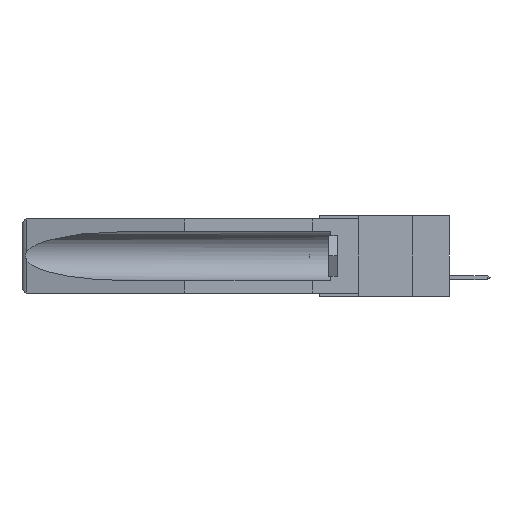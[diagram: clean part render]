
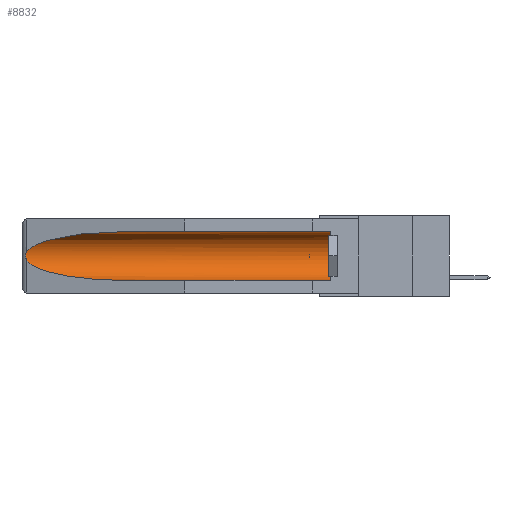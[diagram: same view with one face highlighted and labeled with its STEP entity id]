
A CAD part, left-side view. The second image highlights one B-rep face of the part: STEP entity #8832.
In plain terms, the highlighted cylindrical face has radius 2.857 mm (diameter 5.715 mm), a partial arc.
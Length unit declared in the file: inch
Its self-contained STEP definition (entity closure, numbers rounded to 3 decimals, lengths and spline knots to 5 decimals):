
#994 = ORIENTED_EDGE ( 'NONE', *, *, #16064, .T. ) ;
#1166 = CARTESIAN_POINT ( 'NONE',  ( 0.21114, 1.30732, -0.284 ) ) ;
#1522 = CARTESIAN_POINT ( 'NONE',  ( 0.2675, 1.53308, -0.17534 ) ) ;
#3514 = ORIENTED_EDGE ( 'NONE', *, *, #29029, .T. ) ;
#3515 = CARTESIAN_POINT ( 'NONE',  ( 0.25451, 1.48313, -0.24835 ) ) ;
#3572 = CARTESIAN_POINT ( 'NONE',  ( 0.26537, 1.52718, -0.14972 ) ) ;
#3663 = VERTEX_POINT ( 'NONE', #31776 ) ;
#4320 = CARTESIAN_POINT ( 'NONE',  ( 0.2675, 1.53308, -0.16763 ) ) ;
#4430 = CARTESIAN_POINT ( 'NONE',  ( 0.26597, 1.5296, -0.19026 ) ) ;
#5067 = CARTESIAN_POINT ( 'NONE',  ( 0.155, -0.30754, -0.1715 ) ) ;
#6015 = CARTESIAN_POINT ( 'NONE',  ( 0.155, 1.07973, -0.059 ) ) ;
#6191 = LINE ( 'NONE', #8923, #11631 ) ;
#6878 = CARTESIAN_POINT ( 'NONE',  ( 0.26537, 1.52718, -0.19328 ) ) ;
#7619 = CYLINDRICAL_SURFACE ( 'NONE', #25311, 0.1125 ) ;
#8011 = ORIENTED_EDGE ( 'NONE', *, *, #21563, .F. ) ;
#8250 = CARTESIAN_POINT ( 'NONE',  ( 0.155, 0.126, -0.284 ) ) ;
#8832 = ADVANCED_FACE ( 'NONE', ( #28910 ), #7619, .F. ) ;
#8923 = CARTESIAN_POINT ( 'NONE',  ( 0.155, -0.30754, -0.059 ) ) ;
#9689 = CARTESIAN_POINT ( 'NONE',  ( 0.2673, 1.5327, -0.16383 ) ) ;
#10034 = CARTESIAN_POINT ( 'NONE',  ( 0.26654, 1.53092, -0.15636 ) ) ;
#10948 = CARTESIAN_POINT ( 'NONE',  ( 0.155, -0.30754, -0.284 ) ) ;
#11548 = VERTEX_POINT ( 'NONE', #20221 ) ;
#11631 = VECTOR ( 'NONE', #27247, 39.37008 ) ;
#13234 = B_SPLINE_CURVE_WITH_KNOTS ( 'NONE', 3,
 ( #17983, #25590, #10034, #9689, #4320, #1522, #20552, #17507, #4430, #6878 ),
 .UNSPECIFIED., .F., .F.,
 ( 4, 2, 2, 2, 4 ),
 ( 0., 0.00029, 0.00058, 0.00087, 0.00117 ),
 .UNSPECIFIED. ) ;
#13338 = DIRECTION ( 'NONE',  ( 0., 1., 0. ) ) ;
#13407 = DIRECTION ( 'NONE',  ( 0., 1., 0. ) ) ;
#14192 = CARTESIAN_POINT ( 'NONE',  ( 0.21114, 1.30732, -0.059 ) ) ;
#14549 = VECTOR ( 'NONE', #13407, 39.37008 ) ;
#14840 = CARTESIAN_POINT ( 'NONE',  ( 0.155, 1.07973, -0.284 ) ) ;
#15568 = VERTEX_POINT ( 'NONE', #8250 ) ;
#15584 = DIRECTION ( 'NONE',  ( 0., -1., 0. ) ) ;
#16064 = EDGE_CURVE ( 'NONE', #15568, #30093, #21509, .T. ) ;
#16155 = ORIENTED_EDGE ( 'NONE', *, *, #25836, .T. ) ;
#16664 = LINE ( 'NONE', #10948, #14549 ) ;
#17188 = CARTESIAN_POINT ( 'NONE',  ( 0.26537, 1.52718, -0.19328 ) ) ;
#17507 = CARTESIAN_POINT ( 'NONE',  ( 0.26655, 1.53094, -0.18657 ) ) ;
#17831 = VERTEX_POINT ( 'NONE', #32476 ) ;
#17983 = CARTESIAN_POINT ( 'NONE',  ( 0.26537, 1.52718, -0.14972 ) ) ;
#19095 = EDGE_LOOP ( 'NONE', ( #16155, #22995, #3514, #8011, #994, #25543 ) ) ;
#20221 = CARTESIAN_POINT ( 'NONE',  ( 0.26537, 1.52718, -0.19328 ) ) ;
#20301 = CARTESIAN_POINT ( 'NONE',  ( 0.155, 1.07973, -0.059 ) ) ;
#20552 = CARTESIAN_POINT ( 'NONE',  ( 0.2673, 1.53269, -0.17917 ) ) ;
#21509 = CIRCLE ( 'NONE', #23183, 0.1125 ) ;
#21563 = EDGE_CURVE ( 'NONE', #15568, #17831, #16664, .T. ) ;
#22122 = CARTESIAN_POINT ( 'NONE',  ( 0.25451, 1.48313, -0.09465 ) ) ;
#22635 =( BOUNDED_CURVE ( )  B_SPLINE_CURVE ( 3, ( #17188, #3515, #1166, #14840 ),
 .UNSPECIFIED., .F., .F. ) 
 B_SPLINE_CURVE_WITH_KNOTS ( ( 4, 4 ),
 ( 0.1948, 1.5708 ),
 .UNSPECIFIED. ) 
 CURVE ( )  GEOMETRIC_REPRESENTATION_ITEM ( )  RATIONAL_B_SPLINE_CURVE ( ( 1., 0.848, 0.848, 1. ) ) 
 REPRESENTATION_ITEM ( '' )  );
#22995 = ORIENTED_EDGE ( 'NONE', *, *, #29917, .T. ) ;
#23183 = AXIS2_PLACEMENT_3D ( 'NONE', #31542, #15584, #34198 ) ;
#23717 = VERTEX_POINT ( 'NONE', #20301 ) ;
#23856 = DIRECTION ( 'NONE',  ( 0., 0., 1. ) ) ;
#25311 = AXIS2_PLACEMENT_3D ( 'NONE', #5067, #13338, #23856 ) ;
#25543 = ORIENTED_EDGE ( 'NONE', *, *, #28626, .T. ) ;
#25590 = CARTESIAN_POINT ( 'NONE',  ( 0.26597, 1.52961, -0.15275 ) ) ;
#25836 = EDGE_CURVE ( 'NONE', #23717, #3663, #32432, .T. ) ;
#27247 = DIRECTION ( 'NONE',  ( 0., 1., 0. ) ) ;
#28626 = EDGE_CURVE ( 'NONE', #30093, #23717, #6191, .T. ) ;
#28910 = FACE_OUTER_BOUND ( 'NONE', #19095, .T. ) ;
#28928 = CARTESIAN_POINT ( 'NONE',  ( 0.155, 0.126, -0.059 ) ) ;
#29029 = EDGE_CURVE ( 'NONE', #11548, #17831, #22635, .T. ) ;
#29917 = EDGE_CURVE ( 'NONE', #3663, #11548, #13234, .T. ) ;
#30093 = VERTEX_POINT ( 'NONE', #28928 ) ;
#31542 = CARTESIAN_POINT ( 'NONE',  ( 0.155, 0.126, -0.1715 ) ) ;
#31776 = CARTESIAN_POINT ( 'NONE',  ( 0.26537, 1.52718, -0.14972 ) ) ;
#32432 =( BOUNDED_CURVE ( )  B_SPLINE_CURVE ( 3, ( #6015, #14192, #22122, #3572 ),
 .UNSPECIFIED., .F., .T. ) 
 B_SPLINE_CURVE_WITH_KNOTS ( ( 4, 4 ),
 ( 4.71239, 6.08839 ),
 .UNSPECIFIED. ) 
 CURVE ( )  GEOMETRIC_REPRESENTATION_ITEM ( )  RATIONAL_B_SPLINE_CURVE ( ( 1., 0.848, 0.848, 1. ) ) 
 REPRESENTATION_ITEM ( '' )  );
#32476 = CARTESIAN_POINT ( 'NONE',  ( 0.155, 1.07973, -0.284 ) ) ;
#34198 = DIRECTION ( 'NONE',  ( 0., 0., 1. ) ) ;
